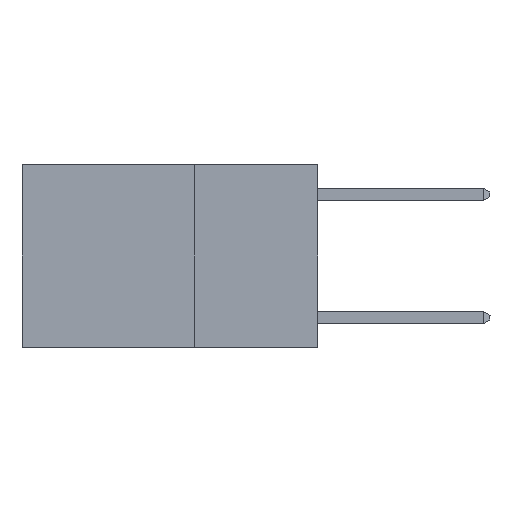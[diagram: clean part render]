
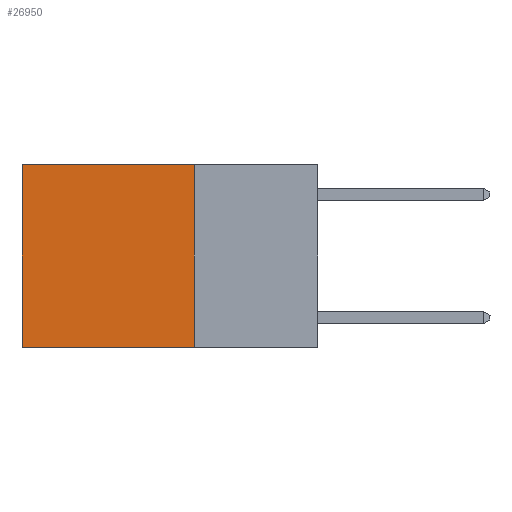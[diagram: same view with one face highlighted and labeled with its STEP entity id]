
A CAD part, left-side view. The second image highlights one B-rep face of the part: STEP entity #26950.
In plain terms, the highlighted planar face has unit normal (-1, 0, 0).
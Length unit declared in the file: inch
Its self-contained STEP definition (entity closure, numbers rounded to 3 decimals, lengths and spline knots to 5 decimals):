
#491 = EDGE_CURVE ( 'NONE', #23860, #7726, #1141, .T. ) ;
#555 = CARTESIAN_POINT ( 'NONE',  ( 0.2625, 0.25, -0.37 ) ) ;
#947 = CARTESIAN_POINT ( 'NONE',  ( 0.2625, 0.6, -0.37 ) ) ;
#1141 = LINE ( 'NONE', #14725, #17050 ) ;
#2401 = CARTESIAN_POINT ( 'NONE',  ( 0.2625, 0.25, 0. ) ) ;
#2958 = DIRECTION ( 'NONE',  ( 0., 0., -1. ) ) ;
#3696 = ORIENTED_EDGE ( 'NONE', *, *, #26233, .T. ) ;
#4526 = PLANE ( 'NONE',  #12192 ) ;
#5026 = VERTEX_POINT ( 'NONE', #11646 ) ;
#7653 = LINE ( 'NONE', #28078, #27074 ) ;
#7726 = VERTEX_POINT ( 'NONE', #555 ) ;
#8102 = DIRECTION ( 'NONE',  ( 0., 1., 0. ) ) ;
#8963 = LINE ( 'NONE', #21373, #22824 ) ;
#9009 = ORIENTED_EDGE ( 'NONE', *, *, #14562, .T. ) ;
#9418 = DIRECTION ( 'NONE',  ( 1., 0., 0. ) ) ;
#9674 = LINE ( 'NONE', #14700, #14888 ) ;
#11646 = CARTESIAN_POINT ( 'NONE',  ( 0.2625, 0.6, 0. ) ) ;
#12192 = AXIS2_PLACEMENT_3D ( 'NONE', #2401, #9418, #2958 ) ;
#14562 = EDGE_CURVE ( 'NONE', #5026, #25614, #7653, .T. ) ;
#14700 = CARTESIAN_POINT ( 'NONE',  ( 0.2625, 0.25, -0.37 ) ) ;
#14725 = CARTESIAN_POINT ( 'NONE',  ( 0.2625, 0.25, 0. ) ) ;
#14888 = VECTOR ( 'NONE', #8102, 39.37008 ) ;
#15287 = DIRECTION ( 'NONE',  ( 0., 0., -1. ) ) ;
#15928 = ORIENTED_EDGE ( 'NONE', *, *, #25121, .F. ) ;
#17050 = VECTOR ( 'NONE', #18885, 39.37008 ) ;
#18885 = DIRECTION ( 'NONE',  ( 0., 0., -1. ) ) ;
#21063 = FACE_OUTER_BOUND ( 'NONE', #23108, .T. ) ;
#21373 = CARTESIAN_POINT ( 'NONE',  ( 0.2625, 0.25, 0. ) ) ;
#22824 = VECTOR ( 'NONE', #23600, 39.37008 ) ;
#23108 = EDGE_LOOP ( 'NONE', ( #9009, #15928, #23161, #3696 ) ) ;
#23161 = ORIENTED_EDGE ( 'NONE', *, *, #491, .F. ) ;
#23600 = DIRECTION ( 'NONE',  ( 0., 1., 0. ) ) ;
#23860 = VERTEX_POINT ( 'NONE', #28601 ) ;
#25121 = EDGE_CURVE ( 'NONE', #7726, #25614, #9674, .T. ) ;
#25614 = VERTEX_POINT ( 'NONE', #947 ) ;
#26233 = EDGE_CURVE ( 'NONE', #23860, #5026, #8963, .T. ) ;
#26950 = ADVANCED_FACE ( 'NONE', ( #21063 ), #4526, .F. ) ;
#27074 = VECTOR ( 'NONE', #15287, 39.37008 ) ;
#28078 = CARTESIAN_POINT ( 'NONE',  ( 0.2625, 0.6, 0. ) ) ;
#28601 = CARTESIAN_POINT ( 'NONE',  ( 0.2625, 0.25, 0. ) ) ;
